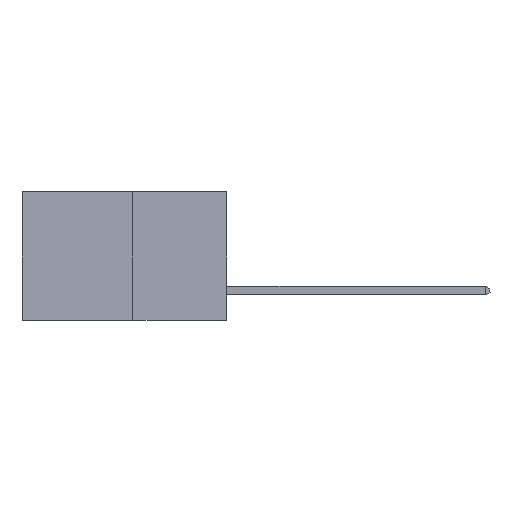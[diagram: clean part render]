
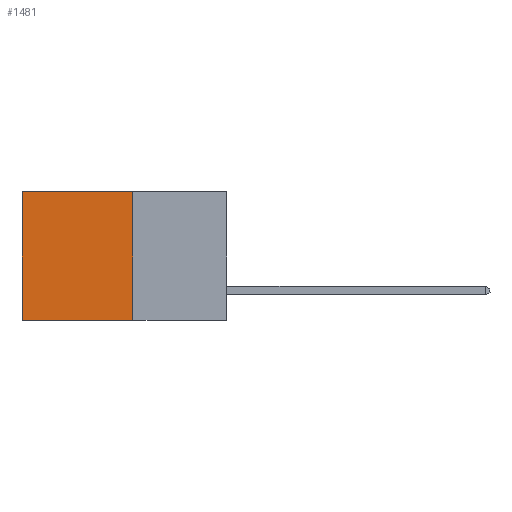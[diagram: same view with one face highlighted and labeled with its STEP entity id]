
A CAD part, left-side view. The second image highlights one B-rep face of the part: STEP entity #1481.
In plain terms, the highlighted planar face has unit normal (-1, 0, 0).
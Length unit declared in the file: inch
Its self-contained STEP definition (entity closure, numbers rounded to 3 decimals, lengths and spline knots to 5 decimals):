
#2 = LINE ( 'NONE', #9785, #972 ) ;
#196 = DIRECTION ( 'NONE',  ( 0., 0., -1. ) ) ;
#313 = DIRECTION ( 'NONE',  ( 0., 1., 0. ) ) ;
#972 = VECTOR ( 'NONE', #313, 39.37008 ) ;
#1369 = CARTESIAN_POINT ( 'NONE',  ( 0.277, 0.59, -0.37 ) ) ;
#1481 = ADVANCED_FACE ( 'NONE', ( #9354 ), #16546, .F. ) ;
#1819 = ORIENTED_EDGE ( 'NONE', *, *, #20282, .T. ) ;
#2101 = VERTEX_POINT ( 'NONE', #7949 ) ;
#2494 = VECTOR ( 'NONE', #196, 39.37008 ) ;
#2970 = DIRECTION ( 'NONE',  ( 0., 0., -1. ) ) ;
#4426 = LINE ( 'NONE', #1369, #16507 ) ;
#4498 = ORIENTED_EDGE ( 'NONE', *, *, #10152, .T. ) ;
#7949 = CARTESIAN_POINT ( 'NONE',  ( 0.277, 0.27, 0. ) ) ;
#8569 = VERTEX_POINT ( 'NONE', #19558 ) ;
#8706 = AXIS2_PLACEMENT_3D ( 'NONE', #16447, #16405, #16343 ) ;
#8860 = CARTESIAN_POINT ( 'NONE',  ( 0.277, 0.59, -0.37 ) ) ;
#8942 = EDGE_CURVE ( 'NONE', #2101, #12119, #18728, .T. ) ;
#9354 = FACE_OUTER_BOUND ( 'NONE', #11508, .T. ) ;
#9785 = CARTESIAN_POINT ( 'NONE',  ( 0.277, 0.27, -0.37 ) ) ;
#9965 = VERTEX_POINT ( 'NONE', #8860 ) ;
#10152 = EDGE_CURVE ( 'NONE', #8569, #9965, #4426, .T. ) ;
#11192 = ORIENTED_EDGE ( 'NONE', *, *, #18133, .F. ) ;
#11508 = EDGE_LOOP ( 'NONE', ( #4498, #11192, #19371, #1819 ) ) ;
#11645 = LINE ( 'NONE', #13433, #19394 ) ;
#12119 = VERTEX_POINT ( 'NONE', #14677 ) ;
#13433 = CARTESIAN_POINT ( 'NONE',  ( 0.277, 0.27, 0. ) ) ;
#14677 = CARTESIAN_POINT ( 'NONE',  ( 0.277, 0.27, -0.37 ) ) ;
#15028 = DIRECTION ( 'NONE',  ( 0., 1., 0. ) ) ;
#16343 = DIRECTION ( 'NONE',  ( 0., 0., -1. ) ) ;
#16405 = DIRECTION ( 'NONE',  ( 1., 0., 0. ) ) ;
#16447 = CARTESIAN_POINT ( 'NONE',  ( 0.277, 0.27, -0.37 ) ) ;
#16507 = VECTOR ( 'NONE', #2970, 39.37008 ) ;
#16546 = PLANE ( 'NONE',  #8706 ) ;
#18133 = EDGE_CURVE ( 'NONE', #12119, #9965, #2, .T. ) ;
#18728 = LINE ( 'NONE', #18998, #2494 ) ;
#18998 = CARTESIAN_POINT ( 'NONE',  ( 0.277, 0.27, -0.37 ) ) ;
#19371 = ORIENTED_EDGE ( 'NONE', *, *, #8942, .F. ) ;
#19394 = VECTOR ( 'NONE', #15028, 39.37008 ) ;
#19558 = CARTESIAN_POINT ( 'NONE',  ( 0.277, 0.59, 0. ) ) ;
#20282 = EDGE_CURVE ( 'NONE', #2101, #8569, #11645, .T. ) ;
